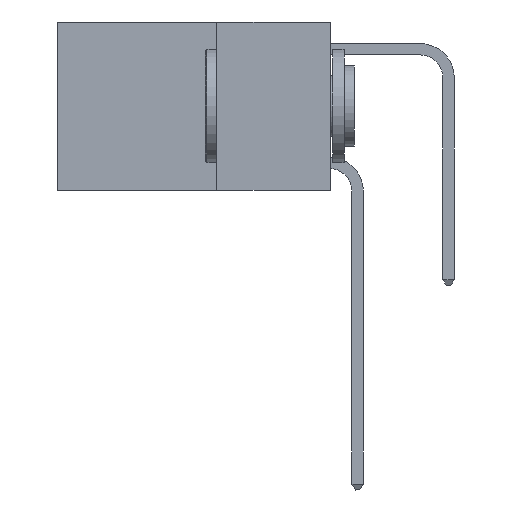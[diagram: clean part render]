
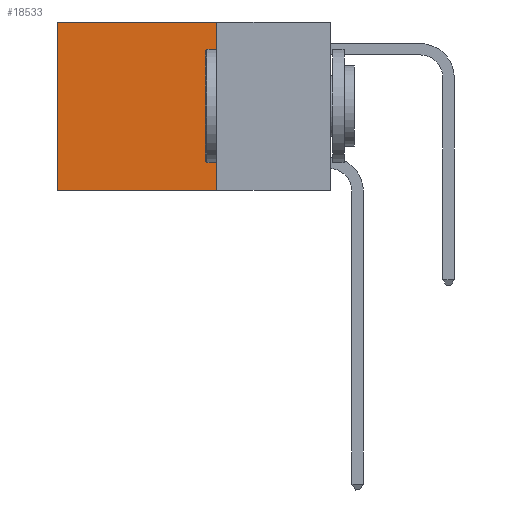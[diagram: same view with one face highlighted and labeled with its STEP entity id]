
A CAD part, left-side view. The second image highlights one B-rep face of the part: STEP entity #18533.
In plain terms, the highlighted planar face has unit normal (-1, 0, 0).
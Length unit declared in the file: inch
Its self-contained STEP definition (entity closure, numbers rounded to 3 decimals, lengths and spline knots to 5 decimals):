
#1119 = VERTEX_POINT ( 'NONE', #10241 ) ;
#2542 = EDGE_CURVE ( 'NONE', #4512, #1119, #20406, .T. ) ;
#2845 = CARTESIAN_POINT ( 'NONE',  ( 0.2625, 0.6, 0. ) ) ;
#3285 = EDGE_CURVE ( 'NONE', #6272, #5118, #5079, .T. ) ;
#3436 = ORIENTED_EDGE ( 'NONE', *, *, #3285, .F. ) ;
#3758 = DIRECTION ( 'NONE',  ( 1., 0., 0. ) ) ;
#3822 = CARTESIAN_POINT ( 'NONE',  ( 0.2625, 0.25, 0. ) ) ;
#4512 = VERTEX_POINT ( 'NONE', #17928 ) ;
#5059 = CARTESIAN_POINT ( 'NONE',  ( 0.2625, 0.6, -0.37 ) ) ;
#5079 = LINE ( 'NONE', #13572, #14988 ) ;
#5118 = VERTEX_POINT ( 'NONE', #5059 ) ;
#5166 = VECTOR ( 'NONE', #9326, 39.37008 ) ;
#5959 = LINE ( 'NONE', #7629, #5166 ) ;
#6272 = VERTEX_POINT ( 'NONE', #9398 ) ;
#7629 = CARTESIAN_POINT ( 'NONE',  ( 0.2625, 0.25, 0. ) ) ;
#8301 = LINE ( 'NONE', #2845, #19225 ) ;
#8811 = EDGE_CURVE ( 'NONE', #4512, #6272, #5959, .T. ) ;
#9326 = DIRECTION ( 'NONE',  ( 0., 0., -1. ) ) ;
#9398 = CARTESIAN_POINT ( 'NONE',  ( 0.2625, 0.25, -0.37 ) ) ;
#10241 = CARTESIAN_POINT ( 'NONE',  ( 0.2625, 0.6, 0. ) ) ;
#10947 = ORIENTED_EDGE ( 'NONE', *, *, #18596, .T. ) ;
#12147 = FACE_OUTER_BOUND ( 'NONE', #14230, .T. ) ;
#12253 = PLANE ( 'NONE',  #14989 ) ;
#13572 = CARTESIAN_POINT ( 'NONE',  ( 0.2625, 0.25, -0.37 ) ) ;
#14230 = EDGE_LOOP ( 'NONE', ( #10947, #3436, #17497, #21920 ) ) ;
#14988 = VECTOR ( 'NONE', #20330, 39.37008 ) ;
#14989 = AXIS2_PLACEMENT_3D ( 'NONE', #19004, #3758, #21550 ) ;
#16758 = DIRECTION ( 'NONE',  ( 0., 0., -1. ) ) ;
#17497 = ORIENTED_EDGE ( 'NONE', *, *, #8811, .F. ) ;
#17928 = CARTESIAN_POINT ( 'NONE',  ( 0.2625, 0.25, 0. ) ) ;
#18437 = VECTOR ( 'NONE', #20302, 39.37008 ) ;
#18533 = ADVANCED_FACE ( 'NONE', ( #12147 ), #12253, .F. ) ;
#18596 = EDGE_CURVE ( 'NONE', #1119, #5118, #8301, .T. ) ;
#19004 = CARTESIAN_POINT ( 'NONE',  ( 0.2625, 0.25, 0. ) ) ;
#19225 = VECTOR ( 'NONE', #16758, 39.37008 ) ;
#20302 = DIRECTION ( 'NONE',  ( 0., 1., 0. ) ) ;
#20330 = DIRECTION ( 'NONE',  ( 0., 1., 0. ) ) ;
#20406 = LINE ( 'NONE', #3822, #18437 ) ;
#21550 = DIRECTION ( 'NONE',  ( 0., 0., -1. ) ) ;
#21920 = ORIENTED_EDGE ( 'NONE', *, *, #2542, .T. ) ;
